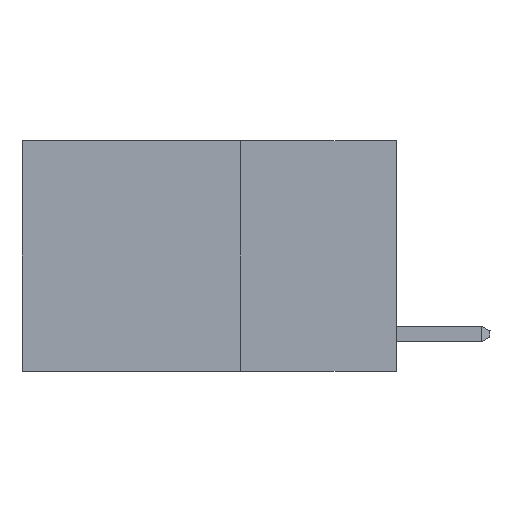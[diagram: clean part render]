
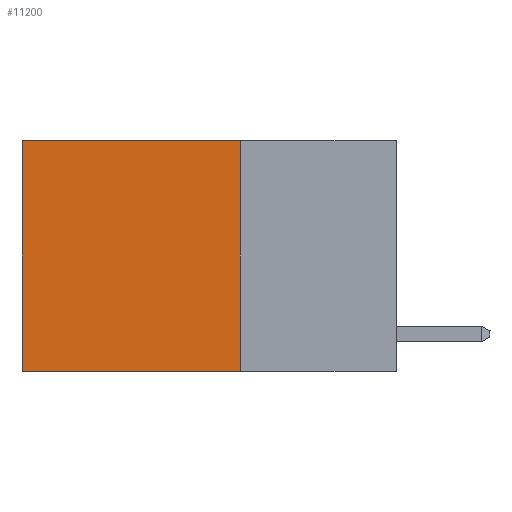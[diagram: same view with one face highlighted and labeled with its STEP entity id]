
A CAD part, left-side view. The second image highlights one B-rep face of the part: STEP entity #11200.
In plain terms, the highlighted planar face has unit normal (-1, 0, 0).
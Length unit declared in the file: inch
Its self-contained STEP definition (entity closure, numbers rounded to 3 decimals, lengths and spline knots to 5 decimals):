
#311 = CARTESIAN_POINT ( 'NONE',  ( 0.2625, 0.6, 0. ) ) ;
#430 = EDGE_CURVE ( 'NONE', #9865, #11422, #11601, .T. ) ;
#1478 = EDGE_CURVE ( 'NONE', #7521, #11422, #14324, .T. ) ;
#3598 = CARTESIAN_POINT ( 'NONE',  ( 0.2625, 0.25, 0. ) ) ;
#4092 = EDGE_CURVE ( 'NONE', #12046, #9865, #10007, .T. ) ;
#5413 = CARTESIAN_POINT ( 'NONE',  ( 0.2625, 0.25, 0. ) ) ;
#5482 = ORIENTED_EDGE ( 'NONE', *, *, #430, .F. ) ;
#5501 = VECTOR ( 'NONE', #11647, 39.37008 ) ;
#6629 = AXIS2_PLACEMENT_3D ( 'NONE', #19167, #13256, #17639 ) ;
#7521 = VERTEX_POINT ( 'NONE', #18710 ) ;
#7980 = EDGE_CURVE ( 'NONE', #12046, #7521, #9702, .T. ) ;
#9087 = ORIENTED_EDGE ( 'NONE', *, *, #1478, .T. ) ;
#9702 = LINE ( 'NONE', #12564, #15980 ) ;
#9865 = VERTEX_POINT ( 'NONE', #10998 ) ;
#10007 = LINE ( 'NONE', #5413, #5501 ) ;
#10998 = CARTESIAN_POINT ( 'NONE',  ( 0.2625, 0.25, -0.37 ) ) ;
#11200 = ADVANCED_FACE ( 'NONE', ( #13351 ), #17742, .F. ) ;
#11422 = VERTEX_POINT ( 'NONE', #16713 ) ;
#11601 = LINE ( 'NONE', #17631, #19955 ) ;
#11647 = DIRECTION ( 'NONE',  ( 0., 0., -1. ) ) ;
#12046 = VERTEX_POINT ( 'NONE', #3598 ) ;
#12564 = CARTESIAN_POINT ( 'NONE',  ( 0.2625, 0.25, 0. ) ) ;
#12787 = DIRECTION ( 'NONE',  ( 0., 0., -1. ) ) ;
#13256 = DIRECTION ( 'NONE',  ( 1., 0., 0. ) ) ;
#13351 = FACE_OUTER_BOUND ( 'NONE', #19610, .T. ) ;
#14324 = LINE ( 'NONE', #311, #14591 ) ;
#14591 = VECTOR ( 'NONE', #12787, 39.37008 ) ;
#14877 = DIRECTION ( 'NONE',  ( 0., 1., 0. ) ) ;
#15980 = VECTOR ( 'NONE', #17061, 39.37008 ) ;
#16713 = CARTESIAN_POINT ( 'NONE',  ( 0.2625, 0.6, -0.37 ) ) ;
#17061 = DIRECTION ( 'NONE',  ( 0., 1., 0. ) ) ;
#17560 = ORIENTED_EDGE ( 'NONE', *, *, #4092, .F. ) ;
#17631 = CARTESIAN_POINT ( 'NONE',  ( 0.2625, 0.25, -0.37 ) ) ;
#17639 = DIRECTION ( 'NONE',  ( 0., 0., -1. ) ) ;
#17742 = PLANE ( 'NONE',  #6629 ) ;
#18676 = ORIENTED_EDGE ( 'NONE', *, *, #7980, .T. ) ;
#18710 = CARTESIAN_POINT ( 'NONE',  ( 0.2625, 0.6, 0. ) ) ;
#19167 = CARTESIAN_POINT ( 'NONE',  ( 0.2625, 0.25, 0. ) ) ;
#19610 = EDGE_LOOP ( 'NONE', ( #9087, #5482, #17560, #18676 ) ) ;
#19955 = VECTOR ( 'NONE', #14877, 39.37008 ) ;
